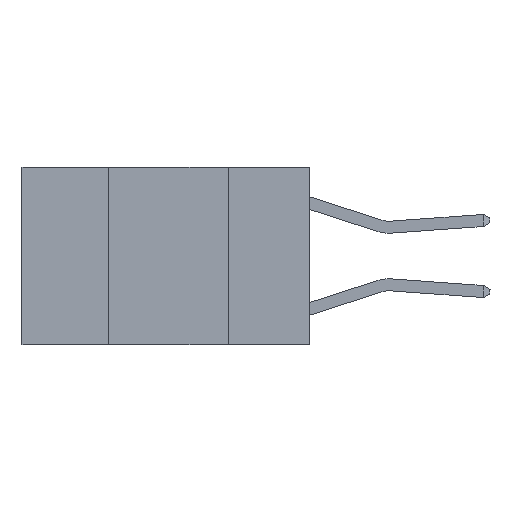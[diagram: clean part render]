
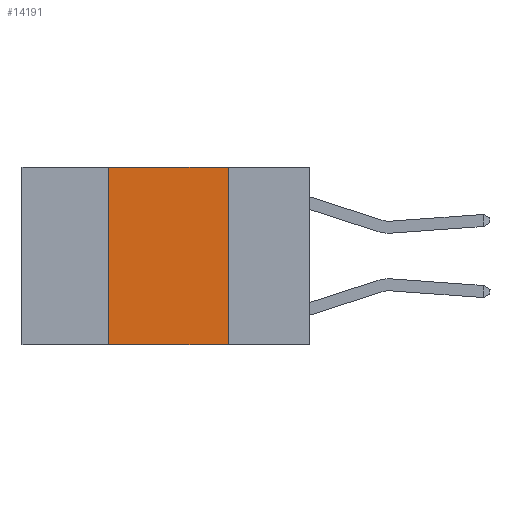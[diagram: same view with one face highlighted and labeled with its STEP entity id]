
A CAD part, left-side view. The second image highlights one B-rep face of the part: STEP entity #14191.
In plain terms, the highlighted planar face has unit normal (-1, 0, 0).
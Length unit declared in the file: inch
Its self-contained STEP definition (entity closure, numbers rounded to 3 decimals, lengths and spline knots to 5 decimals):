
#476 = EDGE_CURVE ( 'NONE', #2599, #9233, #3139, .T. ) ;
#802 = DIRECTION ( 'NONE',  ( 0., 0., -1. ) ) ;
#1711 = CARTESIAN_POINT ( 'NONE',  ( 0., 0.6, 0. ) ) ;
#2448 = AXIS2_PLACEMENT_3D ( 'NONE', #14527, #7640, #802 ) ;
#2588 = DIRECTION ( 'NONE',  ( 0., -1., 0. ) ) ;
#2599 = VERTEX_POINT ( 'NONE', #9824 ) ;
#3139 = LINE ( 'NONE', #9427, #9196 ) ;
#3333 = FACE_OUTER_BOUND ( 'NONE', #8003, .T. ) ;
#4389 = ORIENTED_EDGE ( 'NONE', *, *, #14074, .F. ) ;
#4438 = VERTEX_POINT ( 'NONE', #10928 ) ;
#4969 = CARTESIAN_POINT ( 'NONE',  ( 0., 0.17, 0. ) ) ;
#5098 = ORIENTED_EDGE ( 'NONE', *, *, #476, .T. ) ;
#6185 = DIRECTION ( 'NONE',  ( 0., 0., -1. ) ) ;
#7058 = ORIENTED_EDGE ( 'NONE', *, *, #7651, .F. ) ;
#7640 = DIRECTION ( 'NONE',  ( 1., 0., 0. ) ) ;
#7651 = EDGE_CURVE ( 'NONE', #12928, #9233, #11206, .T. ) ;
#8003 = EDGE_LOOP ( 'NONE', ( #7058, #4389, #10837, #5098 ) ) ;
#8430 = CARTESIAN_POINT ( 'NONE',  ( 0., 0.42, 0. ) ) ;
#8542 = DIRECTION ( 'NONE',  ( 0., -1., 0. ) ) ;
#9196 = VECTOR ( 'NONE', #2588, 39.37008 ) ;
#9233 = VERTEX_POINT ( 'NONE', #11854 ) ;
#9427 = CARTESIAN_POINT ( 'NONE',  ( 0., 0.6, -0.37 ) ) ;
#9824 = CARTESIAN_POINT ( 'NONE',  ( 0., 0.42, -0.37 ) ) ;
#9958 = EDGE_CURVE ( 'NONE', #2599, #4438, #10253, .T. ) ;
#10253 = LINE ( 'NONE', #8430, #12932 ) ;
#10837 = ORIENTED_EDGE ( 'NONE', *, *, #9958, .F. ) ;
#10928 = CARTESIAN_POINT ( 'NONE',  ( 0., 0.42, 0. ) ) ;
#11206 = LINE ( 'NONE', #14200, #14258 ) ;
#11208 = VECTOR ( 'NONE', #8542, 39.37008 ) ;
#11854 = CARTESIAN_POINT ( 'NONE',  ( 0., 0.17, -0.37 ) ) ;
#11890 = DIRECTION ( 'NONE',  ( 0., 0., 1. ) ) ;
#12196 = PLANE ( 'NONE',  #2448 ) ;
#12928 = VERTEX_POINT ( 'NONE', #4969 ) ;
#12932 = VECTOR ( 'NONE', #11890, 39.37008 ) ;
#13891 = LINE ( 'NONE', #1711, #11208 ) ;
#14074 = EDGE_CURVE ( 'NONE', #4438, #12928, #13891, .T. ) ;
#14191 = ADVANCED_FACE ( 'NONE', ( #3333 ), #12196, .F. ) ;
#14200 = CARTESIAN_POINT ( 'NONE',  ( 0., 0.17, 0. ) ) ;
#14258 = VECTOR ( 'NONE', #6185, 39.37008 ) ;
#14527 = CARTESIAN_POINT ( 'NONE',  ( 0., 0.6, 0. ) ) ;
